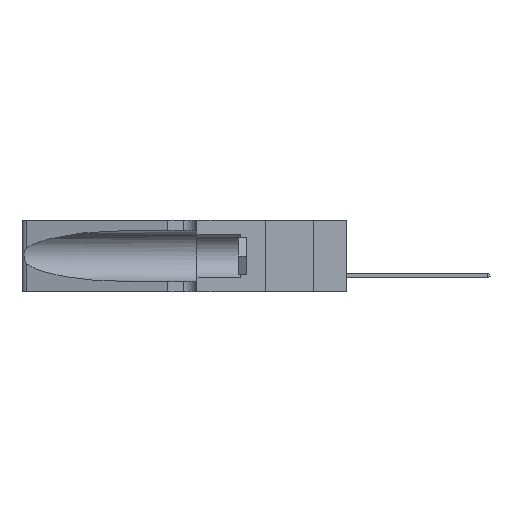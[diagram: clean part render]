
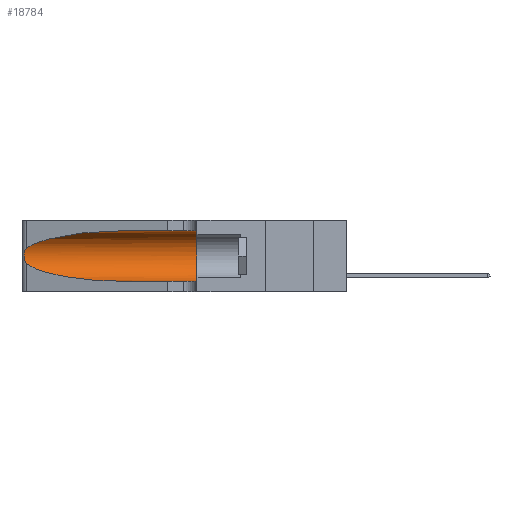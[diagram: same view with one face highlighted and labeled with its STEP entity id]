
A CAD part, left-side view. The second image highlights one B-rep face of the part: STEP entity #18784.
In plain terms, the highlighted cylindrical face has radius 3.308 mm (diameter 6.617 mm), a partial arc.
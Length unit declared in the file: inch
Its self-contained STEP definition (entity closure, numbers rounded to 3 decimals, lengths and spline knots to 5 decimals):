
#178 = VERTEX_POINT ( 'NONE', #364 ) ;
#364 = CARTESIAN_POINT ( 'NONE',  ( 0.25487, 1.22718, 0.22369 ) ) ;
#1795 = EDGE_CURVE ( 'NONE', #28014, #31121, #18748, .T. ) ;
#1883 = CARTESIAN_POINT ( 'NONE',  ( 0.25787, 1.23484, 0.2124 ) ) ;
#1991 = CARTESIAN_POINT ( 'NONE',  ( 0.26017, 1.23833, 0.17102 ) ) ;
#2097 = DIRECTION ( 'NONE',  ( 0., -1., 0. ) ) ;
#2311 = AXIS2_PLACEMENT_3D ( 'NONE', #15474, #15140, #22464 ) ;
#3592 = ORIENTED_EDGE ( 'NONE', *, *, #1795, .T. ) ;
#3639 = CARTESIAN_POINT ( 'NONE',  ( 0.1305, 0.35, 0.05475 ) ) ;
#5941 = CARTESIAN_POINT ( 'NONE',  ( 0.1305, 0.72297, 0.05475 ) ) ;
#6622 = CARTESIAN_POINT ( 'NONE',  ( 0.25639, 1.23184, 0.21858 ) ) ;
#7097 = ORIENTED_EDGE ( 'NONE', *, *, #22514, .T. ) ;
#7610 = B_SPLINE_CURVE_WITH_KNOTS ( 'NONE', 3,
 ( #11605, #31720, #6622, #1883, #24346, #16716, #21579, #19093, #1991, #11711, #26520, #14244, #14550, #16601 ),
 .UNSPECIFIED., .F., .F.,
 ( 4, 2, 2, 2, 2, 2, 4 ),
 ( 0., 0.00027, 0.00053, 0.00107, 0.0016, 0.00187, 0.00214 ),
 .UNSPECIFIED. ) ;
#8142 = LINE ( 'NONE', #14352, #13630 ) ;
#8606 =( BOUNDED_CURVE ( )  B_SPLINE_CURVE ( 3, ( #22164, #24948, #27122, #10010 ),
 .UNSPECIFIED., .F., .T. ) 
 B_SPLINE_CURVE_WITH_KNOTS ( ( 4, 4 ),
 ( 1.5708, 2.84003 ),
 .UNSPECIFIED. ) 
 CURVE ( )  GEOMETRIC_REPRESENTATION_ITEM ( )  RATIONAL_B_SPLINE_CURVE ( ( 1., 0.87, 0.87, 1. ) ) 
 REPRESENTATION_ITEM ( '' )  );
#8660 = VECTOR ( 'NONE', #17819, 39.37008 ) ;
#9758 = CARTESIAN_POINT ( 'NONE',  ( 0.1305, 0.35, 0.31525 ) ) ;
#10010 = CARTESIAN_POINT ( 'NONE',  ( 0.25487, 1.22718, 0.22369 ) ) ;
#10798 = EDGE_CURVE ( 'NONE', #27985, #29168, #14181, .T. ) ;
#11171 = CARTESIAN_POINT ( 'NONE',  ( 0.1305, 0.72297, 0.31525 ) ) ;
#11605 = CARTESIAN_POINT ( 'NONE',  ( 0.25487, 1.22718, 0.22369 ) ) ;
#11711 = CARTESIAN_POINT ( 'NONE',  ( 0.25856, 1.23593, 0.16098 ) ) ;
#13227 = EDGE_CURVE ( 'NONE', #31121, #29168, #8142, .T. ) ;
#13630 = VECTOR ( 'NONE', #2097, 39.37008 ) ;
#14181 = CIRCLE ( 'NONE', #16680, 0.13025 ) ;
#14244 = CARTESIAN_POINT ( 'NONE',  ( 0.25639, 1.23186, 0.15144 ) ) ;
#14352 = CARTESIAN_POINT ( 'NONE',  ( 0.1305, 1.61858, 0.05475 ) ) ;
#14550 = CARTESIAN_POINT ( 'NONE',  ( 0.25555, 1.22993, 0.14849 ) ) ;
#14604 = CARTESIAN_POINT ( 'NONE',  ( 0.1305, 0.35, 0.185 ) ) ;
#15140 = DIRECTION ( 'NONE',  ( 0., -1., 0. ) ) ;
#15474 = CARTESIAN_POINT ( 'NONE',  ( 0.1305, 1.61858, 0.185 ) ) ;
#16072 = LINE ( 'NONE', #17401, #8660 ) ;
#16601 = CARTESIAN_POINT ( 'NONE',  ( 0.25487, 1.22718, 0.14631 ) ) ;
#16652 = ORIENTED_EDGE ( 'NONE', *, *, #25971, .T. ) ;
#16680 = AXIS2_PLACEMENT_3D ( 'NONE', #14604, #23765, #21298 ) ;
#16716 = CARTESIAN_POINT ( 'NONE',  ( 0.26018, 1.23835, 0.19895 ) ) ;
#17401 = CARTESIAN_POINT ( 'NONE',  ( 0.1305, 1.61858, 0.31525 ) ) ;
#17608 = VERTEX_POINT ( 'NONE', #11171 ) ;
#17819 = DIRECTION ( 'NONE',  ( 0., -1., 0. ) ) ;
#18193 = ORIENTED_EDGE ( 'NONE', *, *, #24500, .F. ) ;
#18748 =( BOUNDED_CURVE ( )  B_SPLINE_CURVE ( 3, ( #22274, #29734, #20221, #19904 ),
 .UNSPECIFIED., .F., .T. ) 
 B_SPLINE_CURVE_WITH_KNOTS ( ( 4, 4 ),
 ( 3.44316, 4.71239 ),
 .UNSPECIFIED. ) 
 CURVE ( )  GEOMETRIC_REPRESENTATION_ITEM ( )  RATIONAL_B_SPLINE_CURVE ( ( 1., 0.87, 0.87, 1. ) ) 
 REPRESENTATION_ITEM ( '' )  );
#18784 = ADVANCED_FACE ( 'NONE', ( #28750 ), #20245, .F. ) ;
#19093 = CARTESIAN_POINT ( 'NONE',  ( 0.26075, 1.23896, 0.178 ) ) ;
#19904 = CARTESIAN_POINT ( 'NONE',  ( 0.1305, 0.72297, 0.05475 ) ) ;
#20221 = CARTESIAN_POINT ( 'NONE',  ( 0.18966, 0.96281, 0.05475 ) ) ;
#20245 = CYLINDRICAL_SURFACE ( 'NONE', #2311, 0.13025 ) ;
#21298 = DIRECTION ( 'NONE',  ( 0., 0., 1. ) ) ;
#21579 = CARTESIAN_POINT ( 'NONE',  ( 0.26075, 1.23896, 0.19203 ) ) ;
#22164 = CARTESIAN_POINT ( 'NONE',  ( 0.1305, 0.72297, 0.31525 ) ) ;
#22274 = CARTESIAN_POINT ( 'NONE',  ( 0.25487, 1.22718, 0.14631 ) ) ;
#22464 = DIRECTION ( 'NONE',  ( 0., 0., -1. ) ) ;
#22514 = EDGE_CURVE ( 'NONE', #17608, #178, #8606, .T. ) ;
#23765 = DIRECTION ( 'NONE',  ( 0., 1., 0. ) ) ;
#24346 = CARTESIAN_POINT ( 'NONE',  ( 0.25854, 1.2359, 0.20912 ) ) ;
#24500 = EDGE_CURVE ( 'NONE', #17608, #27985, #16072, .T. ) ;
#24948 = CARTESIAN_POINT ( 'NONE',  ( 0.18966, 0.96281, 0.31525 ) ) ;
#25971 = EDGE_CURVE ( 'NONE', #178, #28014, #7610, .T. ) ;
#26520 = CARTESIAN_POINT ( 'NONE',  ( 0.25789, 1.23486, 0.15765 ) ) ;
#27122 = CARTESIAN_POINT ( 'NONE',  ( 0.2373, 1.15595, 0.28018 ) ) ;
#27957 = EDGE_LOOP ( 'NONE', ( #7097, #16652, #3592, #29182, #29332, #18193 ) ) ;
#27985 = VERTEX_POINT ( 'NONE', #9758 ) ;
#28014 = VERTEX_POINT ( 'NONE', #31598 ) ;
#28750 = FACE_OUTER_BOUND ( 'NONE', #27957, .T. ) ;
#29168 = VERTEX_POINT ( 'NONE', #3639 ) ;
#29182 = ORIENTED_EDGE ( 'NONE', *, *, #13227, .T. ) ;
#29332 = ORIENTED_EDGE ( 'NONE', *, *, #10798, .F. ) ;
#29734 = CARTESIAN_POINT ( 'NONE',  ( 0.2373, 1.15595, 0.08982 ) ) ;
#31121 = VERTEX_POINT ( 'NONE', #5941 ) ;
#31598 = CARTESIAN_POINT ( 'NONE',  ( 0.25487, 1.22718, 0.14631 ) ) ;
#31720 = CARTESIAN_POINT ( 'NONE',  ( 0.25555, 1.22994, 0.2215 ) ) ;
